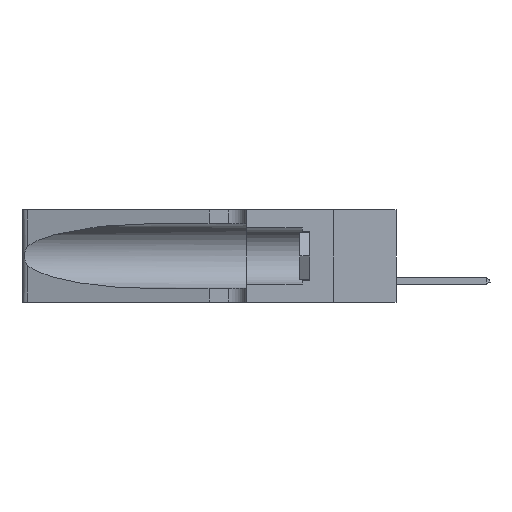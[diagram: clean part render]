
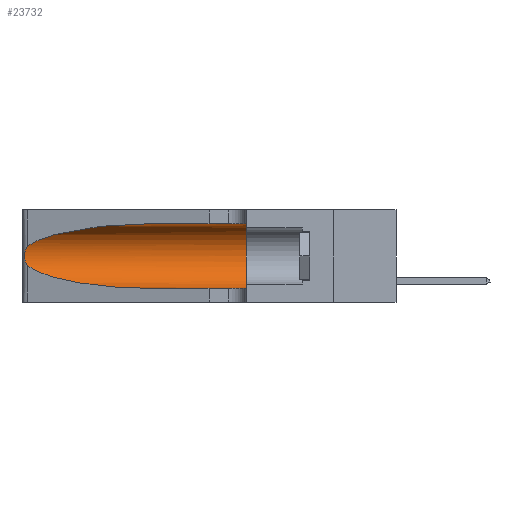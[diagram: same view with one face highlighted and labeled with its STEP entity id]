
A CAD part, left-side view. The second image highlights one B-rep face of the part: STEP entity #23732.
In plain terms, the highlighted cylindrical face has radius 3.308 mm (diameter 6.617 mm), a partial arc.
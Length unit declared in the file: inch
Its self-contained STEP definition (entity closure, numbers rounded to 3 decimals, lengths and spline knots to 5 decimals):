
#770 = EDGE_CURVE ( 'NONE', #4084, #21104, #13867, .T. ) ;
#1309 = ORIENTED_EDGE ( 'NONE', *, *, #770, .F. ) ;
#1335 = CARTESIAN_POINT ( 'NONE',  ( 0.18966, 0.96281, 0.05475 ) ) ;
#1986 = EDGE_LOOP ( 'NONE', ( #36063, #19700, #25583, #45241, #1309, #31383 ) ) ;
#2265 = CARTESIAN_POINT ( 'NONE',  ( 0.25639, 1.23184, 0.21858 ) ) ;
#2799 = CARTESIAN_POINT ( 'NONE',  ( 0.1305, 1.61858, 0.31525 ) ) ;
#4084 = VERTEX_POINT ( 'NONE', #47086 ) ;
#4921 = CARTESIAN_POINT ( 'NONE',  ( 0.25487, 1.22718, 0.14631 ) ) ;
#5257 = CARTESIAN_POINT ( 'NONE',  ( 0.25487, 1.22718, 0.22369 ) ) ;
#5988 =( BOUNDED_CURVE ( )  B_SPLINE_CURVE ( 3, ( #4921, #23707, #1335, #35439 ),
 .UNSPECIFIED., .F., .F. ) 
 B_SPLINE_CURVE_WITH_KNOTS ( ( 4, 4 ),
 ( 3.44316, 4.71239 ),
 .UNSPECIFIED. ) 
 CURVE ( )  GEOMETRIC_REPRESENTATION_ITEM ( )  RATIONAL_B_SPLINE_CURVE ( ( 1., 0.87, 0.87, 1. ) ) 
 REPRESENTATION_ITEM ( '' )  );
#6539 = DIRECTION ( 'NONE',  ( 0., -1., 0. ) ) ;
#7336 = DIRECTION ( 'NONE',  ( 0., 0., -1. ) ) ;
#8060 = VERTEX_POINT ( 'NONE', #9229 ) ;
#8089 = AXIS2_PLACEMENT_3D ( 'NONE', #31209, #24115, #31360 ) ;
#9229 = CARTESIAN_POINT ( 'NONE',  ( 0.25487, 1.22718, 0.14631 ) ) ;
#10515 =( BOUNDED_CURVE ( )  B_SPLINE_CURVE ( 3, ( #14905, #15384, #30306, #14754 ),
 .UNSPECIFIED., .F., .F. ) 
 B_SPLINE_CURVE_WITH_KNOTS ( ( 4, 4 ),
 ( 1.5708, 2.84003 ),
 .UNSPECIFIED. ) 
 CURVE ( )  GEOMETRIC_REPRESENTATION_ITEM ( )  RATIONAL_B_SPLINE_CURVE ( ( 1., 0.87, 0.87, 1. ) ) 
 REPRESENTATION_ITEM ( '' )  );
#11131 = CARTESIAN_POINT ( 'NONE',  ( 0.1305, 0.35, 0.05475 ) ) ;
#12846 = CYLINDRICAL_SURFACE ( 'NONE', #21030, 0.13025 ) ;
#13867 = CIRCLE ( 'NONE', #8089, 0.13025 ) ;
#14754 = CARTESIAN_POINT ( 'NONE',  ( 0.25487, 1.22718, 0.22369 ) ) ;
#14905 = CARTESIAN_POINT ( 'NONE',  ( 0.1305, 0.72297, 0.31525 ) ) ;
#15384 = CARTESIAN_POINT ( 'NONE',  ( 0.18966, 0.96281, 0.31525 ) ) ;
#15730 = FACE_OUTER_BOUND ( 'NONE', #1986, .T. ) ;
#16795 = EDGE_CURVE ( 'NONE', #35386, #8060, #29122, .T. ) ;
#17588 = CARTESIAN_POINT ( 'NONE',  ( 0.25487, 1.22718, 0.22369 ) ) ;
#18077 = CARTESIAN_POINT ( 'NONE',  ( 0.25555, 1.22993, 0.14849 ) ) ;
#19700 = ORIENTED_EDGE ( 'NONE', *, *, #16795, .T. ) ;
#21030 = AXIS2_PLACEMENT_3D ( 'NONE', #24372, #44797, #7336 ) ;
#21104 = VERTEX_POINT ( 'NONE', #11131 ) ;
#21813 = CARTESIAN_POINT ( 'NONE',  ( 0.25487, 1.22718, 0.14631 ) ) ;
#23246 = LINE ( 'NONE', #2799, #35066 ) ;
#23707 = CARTESIAN_POINT ( 'NONE',  ( 0.2373, 1.15595, 0.08982 ) ) ;
#23732 = ADVANCED_FACE ( 'NONE', ( #15730 ), #12846, .F. ) ;
#24115 = DIRECTION ( 'NONE',  ( 0., 1., 0. ) ) ;
#24372 = CARTESIAN_POINT ( 'NONE',  ( 0.1305, 1.61858, 0.185 ) ) ;
#25583 = ORIENTED_EDGE ( 'NONE', *, *, #28591, .T. ) ;
#28591 = EDGE_CURVE ( 'NONE', #8060, #31609, #5988, .T. ) ;
#28953 = CARTESIAN_POINT ( 'NONE',  ( 0.26075, 1.23896, 0.19203 ) ) ;
#29122 = B_SPLINE_CURVE_WITH_KNOTS ( 'NONE', 3,
 ( #17588, #48593, #2265, #43448, #47403, #40173, #28953, #44279, #33233, #33385, #36864, #41142, #18077, #21813 ),
 .UNSPECIFIED., .F., .F.,
 ( 4, 2, 2, 2, 2, 2, 4 ),
 ( 0., 0.00027, 0.00053, 0.00107, 0.0016, 0.00187, 0.00214 ),
 .UNSPECIFIED. ) ;
#30306 = CARTESIAN_POINT ( 'NONE',  ( 0.2373, 1.15595, 0.28018 ) ) ;
#30909 = EDGE_CURVE ( 'NONE', #37187, #4084, #23246, .T. ) ;
#31209 = CARTESIAN_POINT ( 'NONE',  ( 0.1305, 0.35, 0.185 ) ) ;
#31360 = DIRECTION ( 'NONE',  ( 0., 0., 1. ) ) ;
#31383 = ORIENTED_EDGE ( 'NONE', *, *, #30909, .F. ) ;
#31609 = VERTEX_POINT ( 'NONE', #36811 ) ;
#33233 = CARTESIAN_POINT ( 'NONE',  ( 0.26017, 1.23833, 0.17102 ) ) ;
#33385 = CARTESIAN_POINT ( 'NONE',  ( 0.25856, 1.23593, 0.16098 ) ) ;
#33854 = CARTESIAN_POINT ( 'NONE',  ( 0.1305, 0.72297, 0.31525 ) ) ;
#35066 = VECTOR ( 'NONE', #6539, 39.37008 ) ;
#35386 = VERTEX_POINT ( 'NONE', #5257 ) ;
#35439 = CARTESIAN_POINT ( 'NONE',  ( 0.1305, 0.72297, 0.05475 ) ) ;
#36063 = ORIENTED_EDGE ( 'NONE', *, *, #42398, .T. ) ;
#36811 = CARTESIAN_POINT ( 'NONE',  ( 0.1305, 0.72297, 0.05475 ) ) ;
#36864 = CARTESIAN_POINT ( 'NONE',  ( 0.25789, 1.23486, 0.15765 ) ) ;
#37187 = VERTEX_POINT ( 'NONE', #33854 ) ;
#40173 = CARTESIAN_POINT ( 'NONE',  ( 0.26018, 1.23835, 0.19895 ) ) ;
#40860 = DIRECTION ( 'NONE',  ( 0., -1., 0. ) ) ;
#41142 = CARTESIAN_POINT ( 'NONE',  ( 0.25639, 1.23186, 0.15144 ) ) ;
#41333 = CARTESIAN_POINT ( 'NONE',  ( 0.1305, 1.61858, 0.05475 ) ) ;
#41568 = EDGE_CURVE ( 'NONE', #31609, #21104, #45347, .T. ) ;
#42398 = EDGE_CURVE ( 'NONE', #37187, #35386, #10515, .T. ) ;
#42434 = VECTOR ( 'NONE', #40860, 39.37008 ) ;
#43448 = CARTESIAN_POINT ( 'NONE',  ( 0.25787, 1.23484, 0.2124 ) ) ;
#44279 = CARTESIAN_POINT ( 'NONE',  ( 0.26075, 1.23896, 0.178 ) ) ;
#44797 = DIRECTION ( 'NONE',  ( 0., -1., 0. ) ) ;
#45241 = ORIENTED_EDGE ( 'NONE', *, *, #41568, .T. ) ;
#45347 = LINE ( 'NONE', #41333, #42434 ) ;
#47086 = CARTESIAN_POINT ( 'NONE',  ( 0.1305, 0.35, 0.31525 ) ) ;
#47403 = CARTESIAN_POINT ( 'NONE',  ( 0.25854, 1.2359, 0.20912 ) ) ;
#48593 = CARTESIAN_POINT ( 'NONE',  ( 0.25555, 1.22994, 0.2215 ) ) ;
